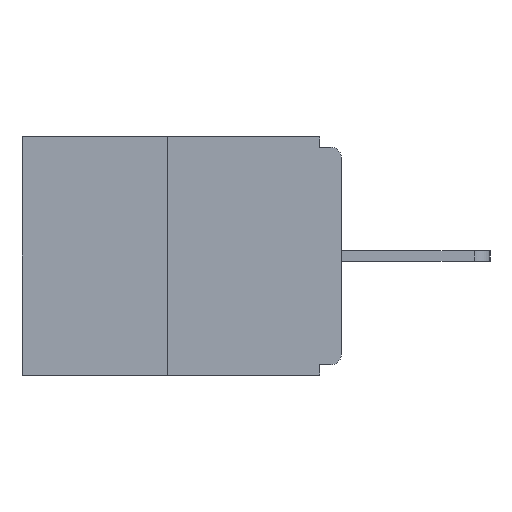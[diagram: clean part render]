
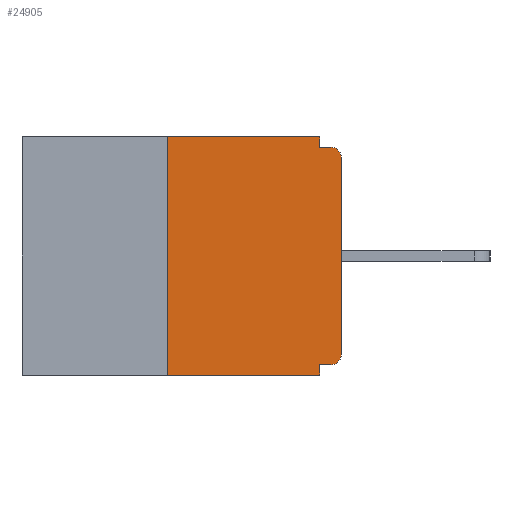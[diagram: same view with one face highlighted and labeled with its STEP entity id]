
A CAD part, left-side view. The second image highlights one B-rep face of the part: STEP entity #24905.
In plain terms, the highlighted planar face has unit normal (-1, 0, 0).
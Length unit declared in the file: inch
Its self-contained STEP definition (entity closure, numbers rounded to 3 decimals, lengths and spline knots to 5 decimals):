
#173 = CARTESIAN_POINT ( 'NONE',  ( 0., 0.015, -0.328 ) ) ;
#193 = VECTOR ( 'NONE', #13154, 39.37008 ) ;
#900 = VERTEX_POINT ( 'NONE', #173 ) ;
#1038 = CIRCLE ( 'NONE', #3901, 0.015 ) ;
#1277 = DIRECTION ( 'NONE',  ( 0., 1., 0. ) ) ;
#1600 = LINE ( 'NONE', #12336, #22238 ) ;
#1742 = VERTEX_POINT ( 'NONE', #9382 ) ;
#1790 = EDGE_CURVE ( 'NONE', #2077, #14785, #20007, .T. ) ;
#1910 = DIRECTION ( 'NONE',  ( 0., 0., 1. ) ) ;
#2077 = VERTEX_POINT ( 'NONE', #22725 ) ;
#2231 = DIRECTION ( 'NONE',  ( 0., 0., -1. ) ) ;
#2494 = EDGE_CURVE ( 'NONE', #19908, #6671, #12186, .T. ) ;
#2610 = LINE ( 'NONE', #3190, #6049 ) ;
#3190 = CARTESIAN_POINT ( 'NONE',  ( 0., 0., -0.328 ) ) ;
#3192 = CARTESIAN_POINT ( 'NONE',  ( 0., 0.25, 0. ) ) ;
#3194 = DIRECTION ( 'NONE',  ( 0., 0., 1. ) ) ;
#3676 = DIRECTION ( 'NONE',  ( 0., -1., 0. ) ) ;
#3850 = CARTESIAN_POINT ( 'NONE',  ( 0., 0.46, -0.343 ) ) ;
#3901 = AXIS2_PLACEMENT_3D ( 'NONE', #5619, #25603, #5527 ) ;
#3946 = LINE ( 'NONE', #14450, #19193 ) ;
#4434 = DIRECTION ( 'NONE',  ( 0., 0., -1. ) ) ;
#4471 = DIRECTION ( 'NONE',  ( 1., 0., 0. ) ) ;
#4719 = CARTESIAN_POINT ( 'NONE',  ( 0., 0.46, 0. ) ) ;
#4933 = ORIENTED_EDGE ( 'NONE', *, *, #2494, .F. ) ;
#5204 = ORIENTED_EDGE ( 'NONE', *, *, #7113, .T. ) ;
#5303 = VECTOR ( 'NONE', #2231, 39.37008 ) ;
#5501 = EDGE_LOOP ( 'NONE', ( #11151, #14879, #5204, #4933, #13450, #5701, #10620, #23722, #14519, #8377 ) ) ;
#5527 = DIRECTION ( 'NONE',  ( 0., 0., -1. ) ) ;
#5619 = CARTESIAN_POINT ( 'NONE',  ( 0., 0.015, -0.313 ) ) ;
#5701 = ORIENTED_EDGE ( 'NONE', *, *, #18357, .T. ) ;
#6049 = VECTOR ( 'NONE', #1277, 39.37008 ) ;
#6671 = VERTEX_POINT ( 'NONE', #13739 ) ;
#7113 = EDGE_CURVE ( 'NONE', #16424, #6671, #24519, .T. ) ;
#8161 = CARTESIAN_POINT ( 'NONE',  ( 0., 0.031, -0.343 ) ) ;
#8377 = ORIENTED_EDGE ( 'NONE', *, *, #12845, .F. ) ;
#8691 = VERTEX_POINT ( 'NONE', #18097 ) ;
#8800 = EDGE_CURVE ( 'NONE', #12319, #14785, #1600, .T. ) ;
#9382 = CARTESIAN_POINT ( 'NONE',  ( 0., 0., -0.313 ) ) ;
#9829 = VECTOR ( 'NONE', #3676, 39.37008 ) ;
#9872 = EDGE_CURVE ( 'NONE', #1742, #2077, #25001, .T. ) ;
#10042 = VECTOR ( 'NONE', #1910, 39.37008 ) ;
#10620 = ORIENTED_EDGE ( 'NONE', *, *, #9872, .T. ) ;
#10926 = CARTESIAN_POINT ( 'NONE',  ( 0., 0.46, 0. ) ) ;
#11144 = CARTESIAN_POINT ( 'NONE',  ( 0., 0.25, 0. ) ) ;
#11151 = ORIENTED_EDGE ( 'NONE', *, *, #13519, .F. ) ;
#12186 = LINE ( 'NONE', #8161, #5303 ) ;
#12298 = VECTOR ( 'NONE', #3194, 39.37008 ) ;
#12319 = VERTEX_POINT ( 'NONE', #16596 ) ;
#12336 = CARTESIAN_POINT ( 'NONE',  ( 0., 0., -0.015 ) ) ;
#12417 = FACE_OUTER_BOUND ( 'NONE', #5501, .T. ) ;
#12508 = DIRECTION ( 'NONE',  ( 0., -1., 0. ) ) ;
#12845 = EDGE_CURVE ( 'NONE', #8691, #12319, #3946, .T. ) ;
#13154 = DIRECTION ( 'NONE',  ( 0., -1., 0. ) ) ;
#13242 = LINE ( 'NONE', #10926, #193 ) ;
#13450 = ORIENTED_EDGE ( 'NONE', *, *, #14615, .F. ) ;
#13519 = EDGE_CURVE ( 'NONE', #24615, #8691, #13242, .T. ) ;
#13739 = CARTESIAN_POINT ( 'NONE',  ( 0., 0.031, -0.343 ) ) ;
#13945 = EDGE_CURVE ( 'NONE', #16424, #24615, #19789, .T. ) ;
#14403 = CARTESIAN_POINT ( 'NONE',  ( 0., 0.25, -0.343 ) ) ;
#14450 = CARTESIAN_POINT ( 'NONE',  ( 0., 0.031, 0. ) ) ;
#14519 = ORIENTED_EDGE ( 'NONE', *, *, #8800, .F. ) ;
#14615 = EDGE_CURVE ( 'NONE', #900, #19908, #2610, .T. ) ;
#14785 = VERTEX_POINT ( 'NONE', #17912 ) ;
#14879 = ORIENTED_EDGE ( 'NONE', *, *, #13945, .F. ) ;
#15723 = CARTESIAN_POINT ( 'NONE',  ( 0., 0.015, -0.03 ) ) ;
#16424 = VERTEX_POINT ( 'NONE', #14403 ) ;
#16596 = CARTESIAN_POINT ( 'NONE',  ( 0., 0.031, -0.015 ) ) ;
#16649 = DIRECTION ( 'NONE',  ( 0., 0., -1. ) ) ;
#17912 = CARTESIAN_POINT ( 'NONE',  ( 0., 0.015, -0.015 ) ) ;
#17935 = CARTESIAN_POINT ( 'NONE',  ( 0., 0., 0. ) ) ;
#18097 = CARTESIAN_POINT ( 'NONE',  ( 0., 0.031, 0. ) ) ;
#18357 = EDGE_CURVE ( 'NONE', #900, #1742, #1038, .T. ) ;
#18856 = AXIS2_PLACEMENT_3D ( 'NONE', #15723, #25540, #25637 ) ;
#19193 = VECTOR ( 'NONE', #4434, 39.37008 ) ;
#19789 = LINE ( 'NONE', #11144, #12298 ) ;
#19908 = VERTEX_POINT ( 'NONE', #20945 ) ;
#20007 = CIRCLE ( 'NONE', #18856, 0.015 ) ;
#20590 = PLANE ( 'NONE',  #21050 ) ;
#20945 = CARTESIAN_POINT ( 'NONE',  ( 0., 0.031, -0.328 ) ) ;
#21050 = AXIS2_PLACEMENT_3D ( 'NONE', #4719, #4471, #16649 ) ;
#22238 = VECTOR ( 'NONE', #12508, 39.37008 ) ;
#22725 = CARTESIAN_POINT ( 'NONE',  ( 0., 0., -0.03 ) ) ;
#23722 = ORIENTED_EDGE ( 'NONE', *, *, #1790, .T. ) ;
#24519 = LINE ( 'NONE', #3850, #9829 ) ;
#24615 = VERTEX_POINT ( 'NONE', #3192 ) ;
#24905 = ADVANCED_FACE ( 'NONE', ( #12417 ), #20590, .F. ) ;
#25001 = LINE ( 'NONE', #17935, #10042 ) ;
#25540 = DIRECTION ( 'NONE',  ( -1., 0., 0. ) ) ;
#25603 = DIRECTION ( 'NONE',  ( -1., 0., 0. ) ) ;
#25637 = DIRECTION ( 'NONE',  ( 0., 0., -1. ) ) ;
